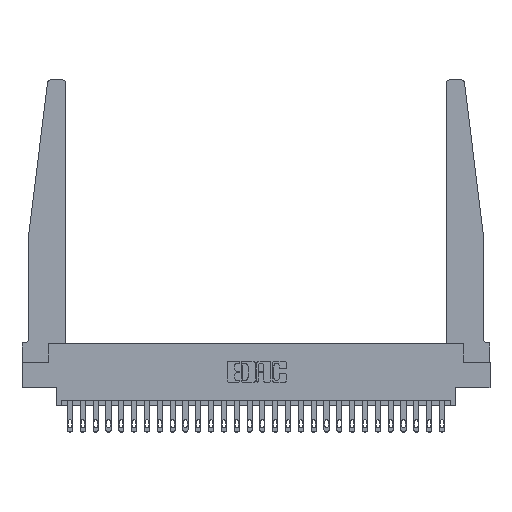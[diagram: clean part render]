
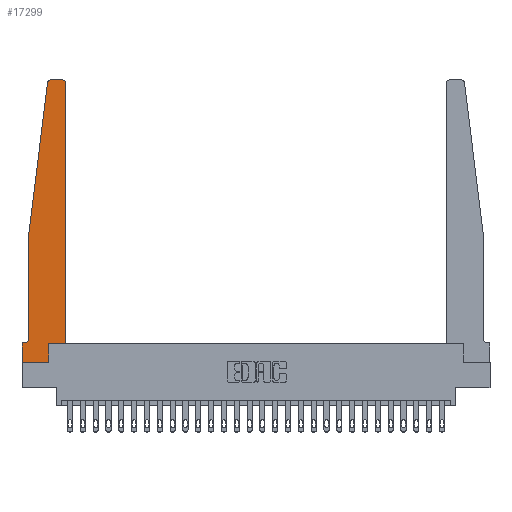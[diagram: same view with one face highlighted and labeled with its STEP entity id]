
A CAD part, top view. The second image highlights one B-rep face of the part: STEP entity #17299.
In plain terms, the highlighted planar face has unit normal (0, 0, 1).
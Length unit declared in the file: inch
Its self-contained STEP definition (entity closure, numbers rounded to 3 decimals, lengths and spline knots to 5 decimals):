
#134 = ORIENTED_EDGE ( 'NONE', *, *, #11428, .T. ) ;
#362 = CARTESIAN_POINT ( 'NONE',  ( 0.27653, 2.72, 0.37 ) ) ;
#456 = LINE ( 'NONE', #14794, #19246 ) ;
#468 = CIRCLE ( 'NONE', #3019, 0.03 ) ;
#580 = DIRECTION ( 'NONE',  ( 0., -1., 0. ) ) ;
#1025 = ORIENTED_EDGE ( 'NONE', *, *, #4229, .T. ) ;
#1077 = VECTOR ( 'NONE', #15882, 39.37008 ) ;
#1554 = EDGE_CURVE ( 'NONE', #10608, #24348, #11032, .T. ) ;
#2145 = CARTESIAN_POINT ( 'NONE',  ( 0.065, 1.25, 0.37 ) ) ;
#2181 = CARTESIAN_POINT ( 'NONE',  ( 0.24675, 2.72367, 0.37 ) ) ;
#2263 = DIRECTION ( 'NONE',  ( 0., 0., 1. ) ) ;
#2498 = CARTESIAN_POINT ( 'NONE',  ( 0., 0., 0.37 ) ) ;
#2775 = AXIS2_PLACEMENT_3D ( 'NONE', #362, #22851, #18586 ) ;
#2828 = ORIENTED_EDGE ( 'NONE', *, *, #7397, .T. ) ;
#3019 = AXIS2_PLACEMENT_3D ( 'NONE', #21435, #25189, #21158 ) ;
#3632 = DIRECTION ( 'NONE',  ( 0., 0., -1. ) ) ;
#4229 = EDGE_CURVE ( 'NONE', #24348, #12085, #12840, .T. ) ;
#4621 = DIRECTION ( 'NONE',  ( 1., 0., 0. ) ) ;
#5192 = EDGE_CURVE ( 'NONE', #6517, #17026, #20498, .T. ) ;
#6167 = VECTOR ( 'NONE', #21736, 39.37008 ) ;
#6219 = EDGE_CURVE ( 'NONE', #8421, #6517, #9172, .T. ) ;
#6259 = PLANE ( 'NONE',  #20495 ) ;
#6517 = VERTEX_POINT ( 'NONE', #18582 ) ;
#6578 = VECTOR ( 'NONE', #11329, 39.37008 ) ;
#6996 = EDGE_CURVE ( 'NONE', #20342, #14640, #456, .T. ) ;
#7116 = CARTESIAN_POINT ( 'NONE',  ( 0.015, 0.1875, 0.37 ) ) ;
#7397 = EDGE_CURVE ( 'NONE', #25743, #8049, #10550, .T. ) ;
#7646 = LINE ( 'NONE', #24132, #6167 ) ;
#7866 = EDGE_CURVE ( 'NONE', #8049, #21433, #14345, .T. ) ;
#8049 = VERTEX_POINT ( 'NONE', #21383 ) ;
#8129 = DIRECTION ( 'NONE',  ( 0., -1., 0. ) ) ;
#8417 = EDGE_LOOP ( 'NONE', ( #2828, #8650, #18112, #22496, #12396, #9897, #23041, #19490, #134, #8577, #1025, #9226 ) ) ;
#8421 = VERTEX_POINT ( 'NONE', #7116 ) ;
#8567 = EDGE_CURVE ( 'NONE', #21433, #20342, #7646, .T. ) ;
#8577 = ORIENTED_EDGE ( 'NONE', *, *, #1554, .T. ) ;
#8650 = ORIENTED_EDGE ( 'NONE', *, *, #7866, .T. ) ;
#9172 = LINE ( 'NONE', #14997, #12777 ) ;
#9226 = ORIENTED_EDGE ( 'NONE', *, *, #21822, .T. ) ;
#9897 = ORIENTED_EDGE ( 'NONE', *, *, #6219, .T. ) ;
#10159 = DIRECTION ( 'NONE',  ( 1., 0., 0. ) ) ;
#10550 = LINE ( 'NONE', #22762, #19149 ) ;
#10608 = VERTEX_POINT ( 'NONE', #23699 ) ;
#11032 = LINE ( 'NONE', #17472, #23568 ) ;
#11329 = DIRECTION ( 'NONE',  ( 0., 1., 0. ) ) ;
#11428 = EDGE_CURVE ( 'NONE', #20835, #10608, #25923, .T. ) ;
#12085 = VERTEX_POINT ( 'NONE', #16744 ) ;
#12396 = ORIENTED_EDGE ( 'NONE', *, *, #24482, .T. ) ;
#12777 = VECTOR ( 'NONE', #25556, 39.37008 ) ;
#12840 = LINE ( 'NONE', #21519, #6578 ) ;
#13182 = DIRECTION ( 'NONE',  ( 1., 0., 0. ) ) ;
#13813 = CIRCLE ( 'NONE', #21926, 0.05 ) ;
#14345 = CIRCLE ( 'NONE', #2775, 0.03 ) ;
#14640 = VERTEX_POINT ( 'NONE', #24032 ) ;
#14732 = DIRECTION ( 'NONE',  ( -1., 0., 0. ) ) ;
#14794 = CARTESIAN_POINT ( 'NONE',  ( 0.065, 1.25, 0.37 ) ) ;
#14997 = CARTESIAN_POINT ( 'NONE',  ( 0.065, 0.1875, 0.37 ) ) ;
#15882 = DIRECTION ( 'NONE',  ( 0., 1., 0. ) ) ;
#16463 = CARTESIAN_POINT ( 'NONE',  ( 0., 0.1875, 0.37 ) ) ;
#16744 = CARTESIAN_POINT ( 'NONE',  ( 0.425, 2.72, 0.37 ) ) ;
#17026 = VERTEX_POINT ( 'NONE', #21209 ) ;
#17299 = ADVANCED_FACE ( 'NONE', ( #24640 ), #6259, .T. ) ;
#17472 = CARTESIAN_POINT ( 'NONE',  ( 0.425, 0.18, 0.37 ) ) ;
#18112 = ORIENTED_EDGE ( 'NONE', *, *, #8567, .T. ) ;
#18582 = CARTESIAN_POINT ( 'NONE',  ( 0., 0.1875, 0.37 ) ) ;
#18586 = DIRECTION ( 'NONE',  ( 1., 0., 0. ) ) ;
#19149 = VECTOR ( 'NONE', #14732, 39.37008 ) ;
#19209 = CARTESIAN_POINT ( 'NONE',  ( 0.395, 2.75, 0.37 ) ) ;
#19246 = VECTOR ( 'NONE', #580, 39.37008 ) ;
#19490 = ORIENTED_EDGE ( 'NONE', *, *, #25814, .T. ) ;
#19884 = VECTOR ( 'NONE', #8129, 39.37008 ) ;
#20007 = DIRECTION ( 'NONE',  ( -1., 0., 0. ) ) ;
#20342 = VERTEX_POINT ( 'NONE', #2145 ) ;
#20350 = VECTOR ( 'NONE', #4621, 39.37008 ) ;
#20495 = AXIS2_PLACEMENT_3D ( 'NONE', #16463, #2263, #10159 ) ;
#20498 = LINE ( 'NONE', #20631, #19884 ) ;
#20544 = CARTESIAN_POINT ( 'NONE',  ( 0.2605, 0.18, 0.37 ) ) ;
#20631 = CARTESIAN_POINT ( 'NONE',  ( 0., 0., 0.37 ) ) ;
#20835 = VERTEX_POINT ( 'NONE', #21429 ) ;
#21158 = DIRECTION ( 'NONE',  ( 1., 0., 0. ) ) ;
#21209 = CARTESIAN_POINT ( 'NONE',  ( 0., 0., 0.37 ) ) ;
#21383 = CARTESIAN_POINT ( 'NONE',  ( 0.27653, 2.75, 0.37 ) ) ;
#21429 = CARTESIAN_POINT ( 'NONE',  ( 0.2605, 0., 0.37 ) ) ;
#21433 = VERTEX_POINT ( 'NONE', #2181 ) ;
#21435 = CARTESIAN_POINT ( 'NONE',  ( 0.395, 2.72, 0.37 ) ) ;
#21519 = CARTESIAN_POINT ( 'NONE',  ( 0.425, 0.18, 0.37 ) ) ;
#21736 = DIRECTION ( 'NONE',  ( -0.122, -0.992, 0. ) ) ;
#21822 = EDGE_CURVE ( 'NONE', #12085, #25743, #468, .T. ) ;
#21926 = AXIS2_PLACEMENT_3D ( 'NONE', #21981, #3632, #20007 ) ;
#21981 = CARTESIAN_POINT ( 'NONE',  ( 0.015, 0.2375, 0.37 ) ) ;
#22496 = ORIENTED_EDGE ( 'NONE', *, *, #6996, .T. ) ;
#22762 = CARTESIAN_POINT ( 'NONE',  ( 0.25, 2.75, 0.37 ) ) ;
#22851 = DIRECTION ( 'NONE',  ( 0., 0., 1. ) ) ;
#23041 = ORIENTED_EDGE ( 'NONE', *, *, #5192, .T. ) ;
#23476 = CARTESIAN_POINT ( 'NONE',  ( 0.425, 0.18, 0.37 ) ) ;
#23568 = VECTOR ( 'NONE', #13182, 39.37008 ) ;
#23699 = CARTESIAN_POINT ( 'NONE',  ( 0.2605, 0.18, 0.37 ) ) ;
#24032 = CARTESIAN_POINT ( 'NONE',  ( 0.065, 0.2375, 0.37 ) ) ;
#24132 = CARTESIAN_POINT ( 'NONE',  ( 0.065, 1.25, 0.37 ) ) ;
#24348 = VERTEX_POINT ( 'NONE', #23476 ) ;
#24482 = EDGE_CURVE ( 'NONE', #14640, #8421, #13813, .T. ) ;
#24640 = FACE_OUTER_BOUND ( 'NONE', #8417, .T. ) ;
#25141 = LINE ( 'NONE', #2498, #20350 ) ;
#25189 = DIRECTION ( 'NONE',  ( 0., 0., 1. ) ) ;
#25556 = DIRECTION ( 'NONE',  ( -1., 0., 0. ) ) ;
#25743 = VERTEX_POINT ( 'NONE', #19209 ) ;
#25814 = EDGE_CURVE ( 'NONE', #17026, #20835, #25141, .T. ) ;
#25923 = LINE ( 'NONE', #20544, #1077 ) ;
